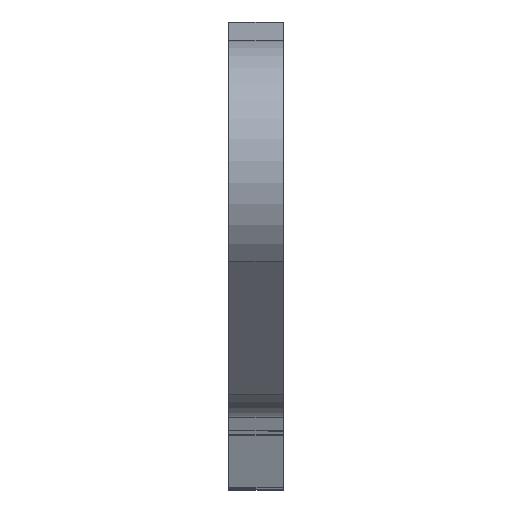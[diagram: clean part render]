
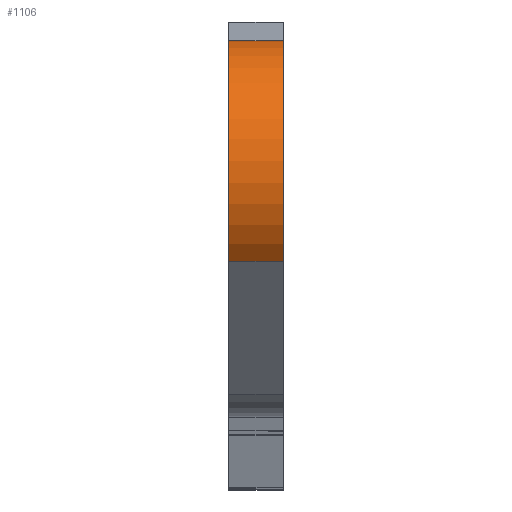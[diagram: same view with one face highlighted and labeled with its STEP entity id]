
A CAD part, top view. The second image highlights one B-rep face of the part: STEP entity #1106.
In plain terms, the highlighted cylindrical face has radius 5.563 mm (diameter 11.125 mm), a partial arc.
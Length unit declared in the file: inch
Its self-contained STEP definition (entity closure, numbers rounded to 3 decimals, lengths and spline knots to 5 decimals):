
#104=FACE_OUTER_BOUND('',#173,.T.);
#173=EDGE_LOOP('',(#877,#878,#879,#880));
#230=CIRCLE('',#1167,0.219);
#235=CIRCLE('',#1179,0.219);
#314=LINE('',#2453,#417);
#318=LINE('',#2487,#421);
#417=VECTOR('',#1318,0.3937);
#421=VECTOR('',#1328,0.3937);
#534=VERTEX_POINT('',#2435);
#535=VERTEX_POINT('',#2437);
#539=VERTEX_POINT('',#2450);
#543=VERTEX_POINT('',#2484);
#649=EDGE_CURVE('',#534,#535,#230,.T.);
#656=EDGE_CURVE('',#539,#534,#314,.T.);
#663=EDGE_CURVE('',#543,#535,#318,.T.);
#666=EDGE_CURVE('',#543,#539,#235,.T.);
#877=ORIENTED_EDGE('',*,*,#666,.F.);
#878=ORIENTED_EDGE('',*,*,#663,.T.);
#879=ORIENTED_EDGE('',*,*,#649,.F.);
#880=ORIENTED_EDGE('',*,*,#656,.F.);
#1072=CYLINDRICAL_SURFACE('',#1178,0.219);
#1106=ADVANCED_FACE('',(#104),#1072,.T.);
#1167=AXIS2_PLACEMENT_3D('',#2438,#1301,#1302);
#1178=AXIS2_PLACEMENT_3D('',#2492,#1333,#1334);
#1179=AXIS2_PLACEMENT_3D('',#2493,#1335,#1336);
#1301=DIRECTION('center_axis',(-1.,0.,0.));
#1302=DIRECTION('ref_axis',(0.,1.,0.));
#1318=DIRECTION('',(-1.,0.,0.));
#1328=DIRECTION('',(-1.,0.,0.));
#1333=DIRECTION('center_axis',(-1.,0.,0.));
#1334=DIRECTION('ref_axis',(0.,1.,0.));
#1335=DIRECTION('center_axis',(1.,0.,0.));
#1336=DIRECTION('ref_axis',(0.,1.,0.));
#2435=CARTESIAN_POINT('',(-0.575,-0.39606,3.42965));
#2437=CARTESIAN_POINT('',(-0.575,-0.031,3.26648));
#2438=CARTESIAN_POINT('Origin',(-0.575,-0.25,3.26648));
#2450=CARTESIAN_POINT('',(-0.485,-0.39606,3.42965));
#2453=CARTESIAN_POINT('',(0.57494,-0.39606,3.42965));
#2484=CARTESIAN_POINT('',(-0.485,-0.031,3.26648));
#2487=CARTESIAN_POINT('',(0.57494,-0.031,3.26648));
#2492=CARTESIAN_POINT('Origin',(0.57494,-0.25,3.26648));
#2493=CARTESIAN_POINT('Origin',(-0.485,-0.25,3.26648));
